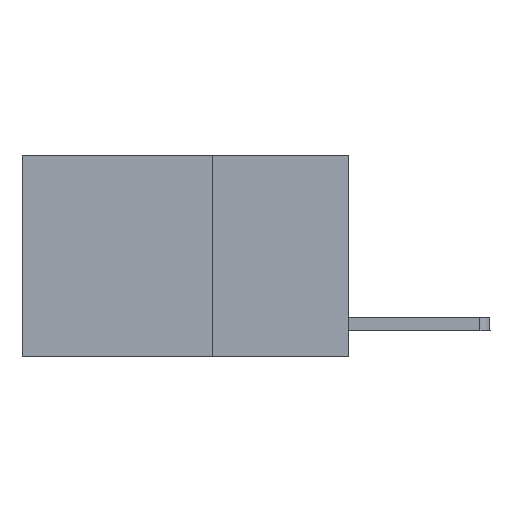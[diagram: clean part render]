
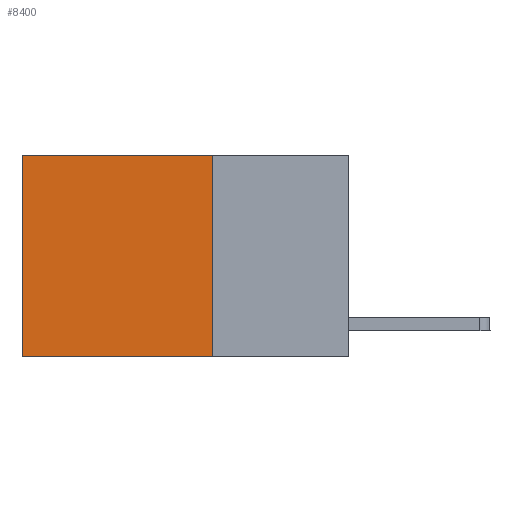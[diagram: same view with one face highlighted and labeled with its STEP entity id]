
A CAD part, left-side view. The second image highlights one B-rep face of the part: STEP entity #8400.
In plain terms, the highlighted planar face has unit normal (-1, 0, 0).
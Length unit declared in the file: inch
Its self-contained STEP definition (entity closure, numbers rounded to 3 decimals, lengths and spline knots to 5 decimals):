
#86 = CARTESIAN_POINT ( 'NONE',  ( 0.2625, 0.25, -0.37 ) ) ;
#1264 = CARTESIAN_POINT ( 'NONE',  ( 0.2625, 0.25, 0. ) ) ;
#1369 = VECTOR ( 'NONE', #9992, 39.37008 ) ;
#1581 = VERTEX_POINT ( 'NONE', #10197 ) ;
#2433 = CARTESIAN_POINT ( 'NONE',  ( 0.2625, 0.25, 0. ) ) ;
#2519 = VERTEX_POINT ( 'NONE', #2433 ) ;
#2611 = CARTESIAN_POINT ( 'NONE',  ( 0.2625, 0.25, 0. ) ) ;
#2633 = ORIENTED_EDGE ( 'NONE', *, *, #3864, .F. ) ;
#2647 = EDGE_LOOP ( 'NONE', ( #5082, #3153, #2633, #9174 ) ) ;
#3153 = ORIENTED_EDGE ( 'NONE', *, *, #7608, .F. ) ;
#3567 = DIRECTION ( 'NONE',  ( 0., 1., 0. ) ) ;
#3864 = EDGE_CURVE ( 'NONE', #2519, #5101, #9886, .T. ) ;
#4751 = DIRECTION ( 'NONE',  ( 1., 0., 0. ) ) ;
#5082 = ORIENTED_EDGE ( 'NONE', *, *, #5956, .T. ) ;
#5101 = VERTEX_POINT ( 'NONE', #7072 ) ;
#5300 = LINE ( 'NONE', #86, #7205 ) ;
#5422 = DIRECTION ( 'NONE',  ( 0., 0., -1. ) ) ;
#5956 = EDGE_CURVE ( 'NONE', #6757, #1581, #8874, .T. ) ;
#6361 = DIRECTION ( 'NONE',  ( 0., 0., -1. ) ) ;
#6499 = VECTOR ( 'NONE', #6361, 39.37008 ) ;
#6757 = VERTEX_POINT ( 'NONE', #7759 ) ;
#7047 = AXIS2_PLACEMENT_3D ( 'NONE', #1264, #4751, #8269 ) ;
#7072 = CARTESIAN_POINT ( 'NONE',  ( 0.2625, 0.25, -0.37 ) ) ;
#7205 = VECTOR ( 'NONE', #3567, 39.37008 ) ;
#7608 = EDGE_CURVE ( 'NONE', #5101, #1581, #5300, .T. ) ;
#7759 = CARTESIAN_POINT ( 'NONE',  ( 0.2625, 0.6, 0. ) ) ;
#8269 = DIRECTION ( 'NONE',  ( 0., 0., -1. ) ) ;
#8400 = ADVANCED_FACE ( 'NONE', ( #9137 ), #10905, .F. ) ;
#8874 = LINE ( 'NONE', #10653, #10775 ) ;
#9112 = EDGE_CURVE ( 'NONE', #2519, #6757, #9238, .T. ) ;
#9137 = FACE_OUTER_BOUND ( 'NONE', #2647, .T. ) ;
#9174 = ORIENTED_EDGE ( 'NONE', *, *, #9112, .T. ) ;
#9238 = LINE ( 'NONE', #10897, #1369 ) ;
#9886 = LINE ( 'NONE', #2611, #6499 ) ;
#9992 = DIRECTION ( 'NONE',  ( 0., 1., 0. ) ) ;
#10197 = CARTESIAN_POINT ( 'NONE',  ( 0.2625, 0.6, -0.37 ) ) ;
#10653 = CARTESIAN_POINT ( 'NONE',  ( 0.2625, 0.6, 0. ) ) ;
#10775 = VECTOR ( 'NONE', #5422, 39.37008 ) ;
#10897 = CARTESIAN_POINT ( 'NONE',  ( 0.2625, 0.25, 0. ) ) ;
#10905 = PLANE ( 'NONE',  #7047 ) ;
